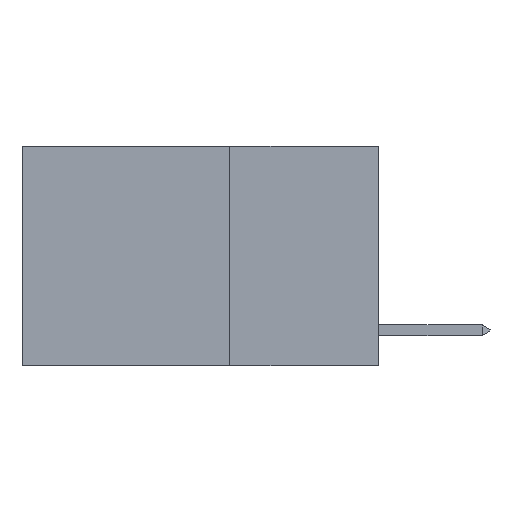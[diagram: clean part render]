
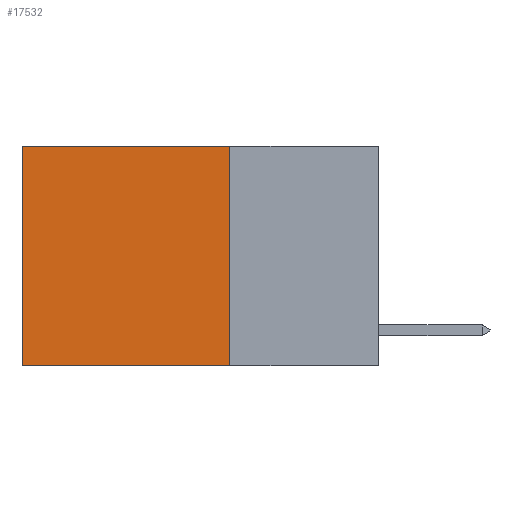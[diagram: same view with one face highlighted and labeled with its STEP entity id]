
A CAD part, left-side view. The second image highlights one B-rep face of the part: STEP entity #17532.
In plain terms, the highlighted planar face has unit normal (-1, 0, 0).
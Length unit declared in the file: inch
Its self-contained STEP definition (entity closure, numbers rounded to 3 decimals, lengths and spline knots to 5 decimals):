
#457 = EDGE_LOOP ( 'NONE', ( #7133, #844, #18371, #9375 ) ) ;
#545 = CARTESIAN_POINT ( 'NONE',  ( 0.2625, 0.25, 0. ) ) ;
#844 = ORIENTED_EDGE ( 'NONE', *, *, #20531, .F. ) ;
#1372 = VECTOR ( 'NONE', #29411, 39.37008 ) ;
#1676 = CARTESIAN_POINT ( 'NONE',  ( 0.2625, 0.25, 0. ) ) ;
#2466 = CARTESIAN_POINT ( 'NONE',  ( 0.2625, 0.6, 0. ) ) ;
#3235 = DIRECTION ( 'NONE',  ( 0., 1., 0. ) ) ;
#3493 = CARTESIAN_POINT ( 'NONE',  ( 0.2625, 0.25, 0. ) ) ;
#5813 = DIRECTION ( 'NONE',  ( 1., 0., 0. ) ) ;
#6466 = CARTESIAN_POINT ( 'NONE',  ( 0.2625, 0.25, 0. ) ) ;
#6849 = FACE_OUTER_BOUND ( 'NONE', #457, .T. ) ;
#6887 = VERTEX_POINT ( 'NONE', #1676 ) ;
#7133 = ORIENTED_EDGE ( 'NONE', *, *, #17245, .T. ) ;
#8409 = CARTESIAN_POINT ( 'NONE',  ( 0.2625, 0.6, 0. ) ) ;
#8633 = LINE ( 'NONE', #2466, #13999 ) ;
#8874 = VECTOR ( 'NONE', #18986, 39.37008 ) ;
#9254 = AXIS2_PLACEMENT_3D ( 'NONE', #3493, #5813, #21868 ) ;
#9375 = ORIENTED_EDGE ( 'NONE', *, *, #27063, .T. ) ;
#9447 = CARTESIAN_POINT ( 'NONE',  ( 0.2625, 0.25, -0.37 ) ) ;
#10807 = VERTEX_POINT ( 'NONE', #8409 ) ;
#11919 = CARTESIAN_POINT ( 'NONE',  ( 0.2625, 0.6, -0.37 ) ) ;
#13670 = LINE ( 'NONE', #6466, #1372 ) ;
#13999 = VECTOR ( 'NONE', #27715, 39.37008 ) ;
#17065 = EDGE_CURVE ( 'NONE', #6887, #17844, #13670, .T. ) ;
#17081 = VECTOR ( 'NONE', #3235, 39.37008 ) ;
#17245 = EDGE_CURVE ( 'NONE', #10807, #23163, #8633, .T. ) ;
#17532 = ADVANCED_FACE ( 'NONE', ( #6849 ), #19567, .F. ) ;
#17844 = VERTEX_POINT ( 'NONE', #9447 ) ;
#18371 = ORIENTED_EDGE ( 'NONE', *, *, #17065, .F. ) ;
#18986 = DIRECTION ( 'NONE',  ( 0., 1., 0. ) ) ;
#19311 = CARTESIAN_POINT ( 'NONE',  ( 0.2625, 0.25, -0.37 ) ) ;
#19567 = PLANE ( 'NONE',  #9254 ) ;
#20531 = EDGE_CURVE ( 'NONE', #17844, #23163, #29316, .T. ) ;
#21868 = DIRECTION ( 'NONE',  ( 0., 0., -1. ) ) ;
#23163 = VERTEX_POINT ( 'NONE', #11919 ) ;
#27063 = EDGE_CURVE ( 'NONE', #6887, #10807, #27895, .T. ) ;
#27715 = DIRECTION ( 'NONE',  ( 0., 0., -1. ) ) ;
#27895 = LINE ( 'NONE', #545, #8874 ) ;
#29316 = LINE ( 'NONE', #19311, #17081 ) ;
#29411 = DIRECTION ( 'NONE',  ( 0., 0., -1. ) ) ;
